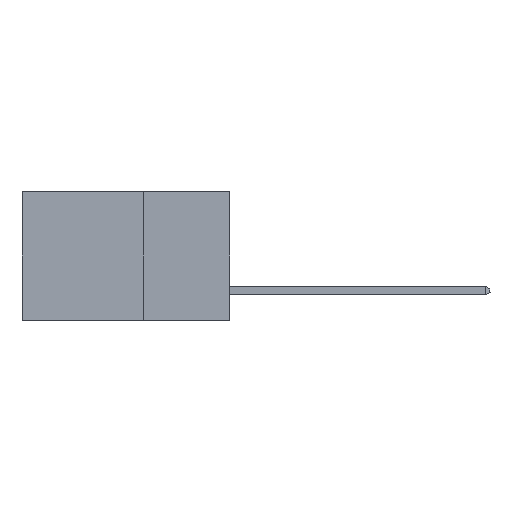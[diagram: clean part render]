
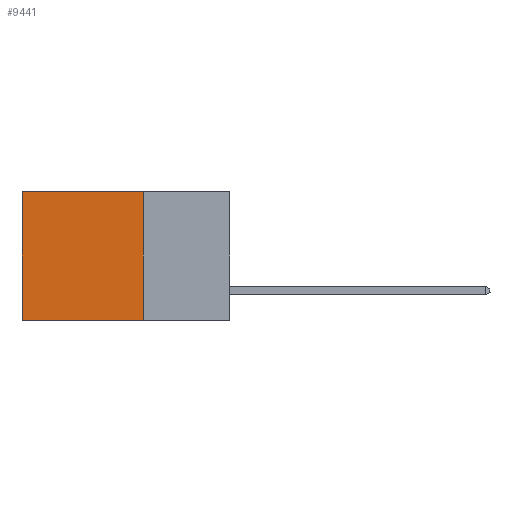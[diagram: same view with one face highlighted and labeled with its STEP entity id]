
A CAD part, left-side view. The second image highlights one B-rep face of the part: STEP entity #9441.
In plain terms, the highlighted planar face has unit normal (-1, 0, 0).
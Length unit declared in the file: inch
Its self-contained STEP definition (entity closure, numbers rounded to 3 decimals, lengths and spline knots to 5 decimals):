
#509 = CARTESIAN_POINT ( 'NONE',  ( 0.298, 0.25, 0. ) ) ;
#735 = VECTOR ( 'NONE', #900, 39.37008 ) ;
#900 = DIRECTION ( 'NONE',  ( 0., 0., -1. ) ) ;
#923 = CARTESIAN_POINT ( 'NONE',  ( 0.298, 0.6, -0.37 ) ) ;
#1329 = VECTOR ( 'NONE', #4999, 39.37008 ) ;
#1569 = DIRECTION ( 'NONE',  ( 0., 0., -1. ) ) ;
#1973 = AXIS2_PLACEMENT_3D ( 'NONE', #10604, #11524, #2220 ) ;
#2022 = CARTESIAN_POINT ( 'NONE',  ( 0.298, 0.25, -0.37 ) ) ;
#2064 = EDGE_CURVE ( 'NONE', #5556, #4949, #8943, .T. ) ;
#2220 = DIRECTION ( 'NONE',  ( 0., 0., -1. ) ) ;
#2260 = ORIENTED_EDGE ( 'NONE', *, *, #3912, .T. ) ;
#2342 = LINE ( 'NONE', #2499, #735 ) ;
#2499 = CARTESIAN_POINT ( 'NONE',  ( 0.298, 0.6, 0. ) ) ;
#3089 = VECTOR ( 'NONE', #7486, 39.37008 ) ;
#3889 = CARTESIAN_POINT ( 'NONE',  ( 0.298, 0.25, -0.37 ) ) ;
#3912 = EDGE_CURVE ( 'NONE', #4949, #8565, #2342, .T. ) ;
#4949 = VERTEX_POINT ( 'NONE', #6014 ) ;
#4993 = ORIENTED_EDGE ( 'NONE', *, *, #12079, .F. ) ;
#4999 = DIRECTION ( 'NONE',  ( 0., 1., 0. ) ) ;
#5556 = VERTEX_POINT ( 'NONE', #5953 ) ;
#5953 = CARTESIAN_POINT ( 'NONE',  ( 0.298, 0.25, 0. ) ) ;
#6014 = CARTESIAN_POINT ( 'NONE',  ( 0.298, 0.6, 0. ) ) ;
#6432 = FACE_OUTER_BOUND ( 'NONE', #7494, .T. ) ;
#6589 = VECTOR ( 'NONE', #1569, 39.37008 ) ;
#6888 = PLANE ( 'NONE',  #1973 ) ;
#6894 = CARTESIAN_POINT ( 'NONE',  ( 0.298, 0.25, 0. ) ) ;
#7279 = LINE ( 'NONE', #3889, #3089 ) ;
#7486 = DIRECTION ( 'NONE',  ( 0., 1., 0. ) ) ;
#7494 = EDGE_LOOP ( 'NONE', ( #2260, #4993, #10236, #12138 ) ) ;
#8384 = LINE ( 'NONE', #509, #6589 ) ;
#8565 = VERTEX_POINT ( 'NONE', #923 ) ;
#8943 = LINE ( 'NONE', #6894, #1329 ) ;
#9441 = ADVANCED_FACE ( 'NONE', ( #6432 ), #6888, .F. ) ;
#10236 = ORIENTED_EDGE ( 'NONE', *, *, #10644, .F. ) ;
#10604 = CARTESIAN_POINT ( 'NONE',  ( 0.298, 0.25, 0. ) ) ;
#10644 = EDGE_CURVE ( 'NONE', #5556, #11319, #8384, .T. ) ;
#11319 = VERTEX_POINT ( 'NONE', #2022 ) ;
#11524 = DIRECTION ( 'NONE',  ( 1., 0., 0. ) ) ;
#12079 = EDGE_CURVE ( 'NONE', #11319, #8565, #7279, .T. ) ;
#12138 = ORIENTED_EDGE ( 'NONE', *, *, #2064, .T. ) ;
